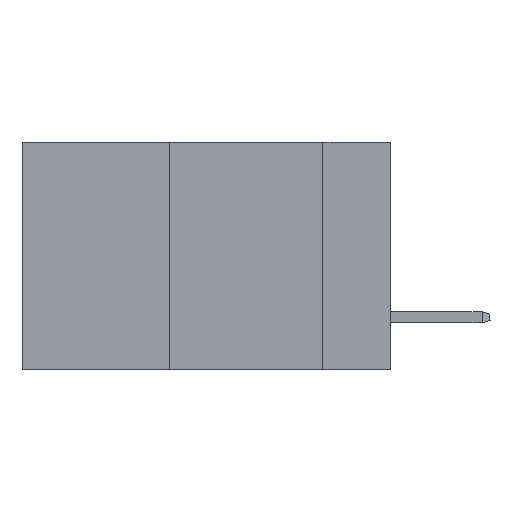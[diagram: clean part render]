
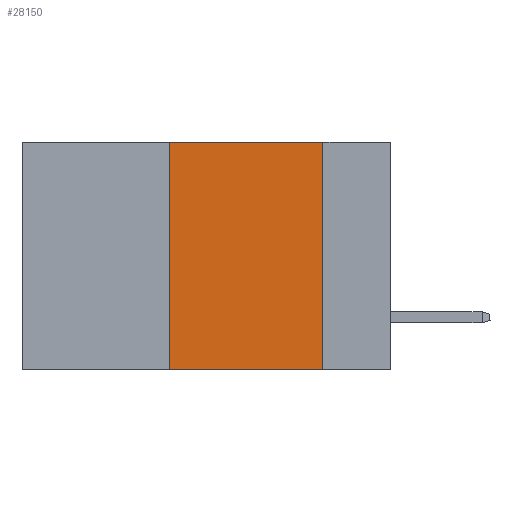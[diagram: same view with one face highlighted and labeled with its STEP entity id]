
A CAD part, left-side view. The second image highlights one B-rep face of the part: STEP entity #28150.
In plain terms, the highlighted planar face has unit normal (-1, 0, 0).
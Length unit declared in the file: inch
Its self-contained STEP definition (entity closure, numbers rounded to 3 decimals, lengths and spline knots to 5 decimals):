
#282 = VERTEX_POINT ( 'NONE', #6745 ) ;
#2718 = EDGE_LOOP ( 'NONE', ( #31451, #15480, #17404, #6260 ) ) ;
#2975 = CARTESIAN_POINT ( 'NONE',  ( 0., 0.6, 0. ) ) ;
#4242 = VECTOR ( 'NONE', #29231, 39.37008 ) ;
#4947 = CARTESIAN_POINT ( 'NONE',  ( 0., 0.36, 0. ) ) ;
#5310 = VERTEX_POINT ( 'NONE', #10074 ) ;
#5791 = LINE ( 'NONE', #4947, #4242 ) ;
#6260 = ORIENTED_EDGE ( 'NONE', *, *, #17355, .T. ) ;
#6745 = CARTESIAN_POINT ( 'NONE',  ( 0., 0.11, 0. ) ) ;
#7432 = DIRECTION ( 'NONE',  ( 1., 0., 0. ) ) ;
#8063 = LINE ( 'NONE', #25491, #26903 ) ;
#8381 = LINE ( 'NONE', #24209, #18038 ) ;
#9776 = VERTEX_POINT ( 'NONE', #27586 ) ;
#10074 = CARTESIAN_POINT ( 'NONE',  ( 0., 0.36, 0. ) ) ;
#11707 = VERTEX_POINT ( 'NONE', #15610 ) ;
#15294 = EDGE_CURVE ( 'NONE', #5310, #282, #25932, .T. ) ;
#15480 = ORIENTED_EDGE ( 'NONE', *, *, #15294, .F. ) ;
#15610 = CARTESIAN_POINT ( 'NONE',  ( 0., 0.11, -0.37 ) ) ;
#17355 = EDGE_CURVE ( 'NONE', #9776, #11707, #8381, .T. ) ;
#17404 = ORIENTED_EDGE ( 'NONE', *, *, #22319, .F. ) ;
#17680 = PLANE ( 'NONE',  #27539 ) ;
#17952 = CARTESIAN_POINT ( 'NONE',  ( 0., 0.6, 0. ) ) ;
#18038 = VECTOR ( 'NONE', #31682, 39.37008 ) ;
#18736 = FACE_OUTER_BOUND ( 'NONE', #2718, .T. ) ;
#22319 = EDGE_CURVE ( 'NONE', #9776, #5310, #5791, .T. ) ;
#24209 = CARTESIAN_POINT ( 'NONE',  ( 0., 0.6, -0.37 ) ) ;
#25150 = VECTOR ( 'NONE', #30098, 39.37008 ) ;
#25491 = CARTESIAN_POINT ( 'NONE',  ( 0., 0.11, 0. ) ) ;
#25932 = LINE ( 'NONE', #17952, #25150 ) ;
#26576 = EDGE_CURVE ( 'NONE', #282, #11707, #8063, .T. ) ;
#26903 = VECTOR ( 'NONE', #27997, 39.37008 ) ;
#27539 = AXIS2_PLACEMENT_3D ( 'NONE', #2975, #7432, #29698 ) ;
#27586 = CARTESIAN_POINT ( 'NONE',  ( 0., 0.36, -0.37 ) ) ;
#27997 = DIRECTION ( 'NONE',  ( 0., 0., -1. ) ) ;
#28150 = ADVANCED_FACE ( 'NONE', ( #18736 ), #17680, .F. ) ;
#29231 = DIRECTION ( 'NONE',  ( 0., 0., 1. ) ) ;
#29698 = DIRECTION ( 'NONE',  ( 0., 0., -1. ) ) ;
#30098 = DIRECTION ( 'NONE',  ( 0., -1., 0. ) ) ;
#31451 = ORIENTED_EDGE ( 'NONE', *, *, #26576, .F. ) ;
#31682 = DIRECTION ( 'NONE',  ( 0., -1., 0. ) ) ;
